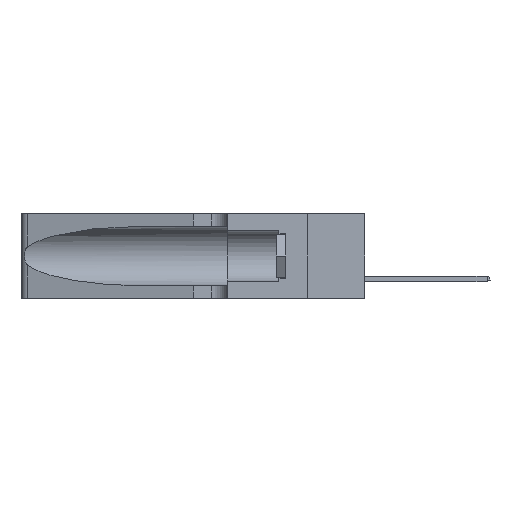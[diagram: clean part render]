
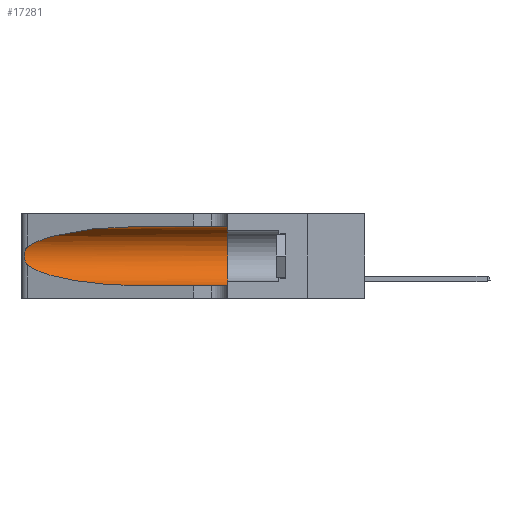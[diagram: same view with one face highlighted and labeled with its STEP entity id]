
A CAD part, left-side view. The second image highlights one B-rep face of the part: STEP entity #17281.
In plain terms, the highlighted cylindrical face has radius 3.308 mm (diameter 6.617 mm), a partial arc.
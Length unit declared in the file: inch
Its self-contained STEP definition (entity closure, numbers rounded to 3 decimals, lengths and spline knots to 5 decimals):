
#176 = CARTESIAN_POINT ( 'NONE',  ( 0.1305, 0.35, 0.31525 ) ) ;
#486 = CARTESIAN_POINT ( 'NONE',  ( 0.26075, 1.23896, 0.178 ) ) ;
#702 = DIRECTION ( 'NONE',  ( 0., -1., 0. ) ) ;
#1172 = VERTEX_POINT ( 'NONE', #8161 ) ;
#1395 = DIRECTION ( 'NONE',  ( 0., -1., 0. ) ) ;
#2424 = VERTEX_POINT ( 'NONE', #16003 ) ;
#2912 = CARTESIAN_POINT ( 'NONE',  ( 0.1305, 0.35, 0.185 ) ) ;
#2987 = DIRECTION ( 'NONE',  ( 0., 1., 0. ) ) ;
#3021 = EDGE_LOOP ( 'NONE', ( #21100, #21108, #21686, #7872, #3442, #13311 ) ) ;
#3167 = B_SPLINE_CURVE_WITH_KNOTS ( 'NONE', 3,
 ( #6841, #21973, #16844, #6610, #8393, #9002, #6990, #486, #12153, #18927, #12298, #3888, #5388, #3669 ),
 .UNSPECIFIED., .F., .F.,
 ( 4, 2, 2, 2, 2, 2, 4 ),
 ( 0., 0.00027, 0.00053, 0.00107, 0.0016, 0.00187, 0.00214 ),
 .UNSPECIFIED. ) ;
#3442 = ORIENTED_EDGE ( 'NONE', *, *, #21819, .F. ) ;
#3669 = CARTESIAN_POINT ( 'NONE',  ( 0.25487, 1.22718, 0.14631 ) ) ;
#3676 = LINE ( 'NONE', #10855, #13487 ) ;
#3888 = CARTESIAN_POINT ( 'NONE',  ( 0.25639, 1.23186, 0.15144 ) ) ;
#3994 = CARTESIAN_POINT ( 'NONE',  ( 0.1305, 0.35, 0.05475 ) ) ;
#4437 = CARTESIAN_POINT ( 'NONE',  ( 0.1305, 0.72297, 0.05475 ) ) ;
#5388 = CARTESIAN_POINT ( 'NONE',  ( 0.25555, 1.22993, 0.14849 ) ) ;
#6610 = CARTESIAN_POINT ( 'NONE',  ( 0.25787, 1.23484, 0.2124 ) ) ;
#6841 = CARTESIAN_POINT ( 'NONE',  ( 0.25487, 1.22718, 0.22369 ) ) ;
#6990 = CARTESIAN_POINT ( 'NONE',  ( 0.26075, 1.23896, 0.19203 ) ) ;
#7119 =( BOUNDED_CURVE ( )  B_SPLINE_CURVE ( 3, ( #11892, #20530, #12055, #13369 ),
 .UNSPECIFIED., .F., .F. ) 
 B_SPLINE_CURVE_WITH_KNOTS ( ( 4, 4 ),
 ( 1.5708, 2.84003 ),
 .UNSPECIFIED. ) 
 CURVE ( )  GEOMETRIC_REPRESENTATION_ITEM ( )  RATIONAL_B_SPLINE_CURVE ( ( 1., 0.87, 0.87, 1. ) ) 
 REPRESENTATION_ITEM ( '' )  );
#7872 = ORIENTED_EDGE ( 'NONE', *, *, #10670, .T. ) ;
#8161 = CARTESIAN_POINT ( 'NONE',  ( 0.25487, 1.22718, 0.14631 ) ) ;
#8183 = CARTESIAN_POINT ( 'NONE',  ( 0.1305, 0.72297, 0.05475 ) ) ;
#8306 = CYLINDRICAL_SURFACE ( 'NONE', #20213, 0.13025 ) ;
#8339 = CARTESIAN_POINT ( 'NONE',  ( 0.1305, 1.61858, 0.185 ) ) ;
#8393 = CARTESIAN_POINT ( 'NONE',  ( 0.25854, 1.2359, 0.20912 ) ) ;
#8400 = CARTESIAN_POINT ( 'NONE',  ( 0.1305, 1.61858, 0.31525 ) ) ;
#8554 = AXIS2_PLACEMENT_3D ( 'NONE', #2912, #2987, #9671 ) ;
#8662 = LINE ( 'NONE', #8400, #20664 ) ;
#8857 = FACE_OUTER_BOUND ( 'NONE', #3021, .T. ) ;
#9002 = CARTESIAN_POINT ( 'NONE',  ( 0.26018, 1.23835, 0.19895 ) ) ;
#9671 = DIRECTION ( 'NONE',  ( 0., 0., 1. ) ) ;
#10670 = EDGE_CURVE ( 'NONE', #20775, #20023, #3676, .T. ) ;
#10855 = CARTESIAN_POINT ( 'NONE',  ( 0.1305, 1.61858, 0.05475 ) ) ;
#11100 =( BOUNDED_CURVE ( )  B_SPLINE_CURVE ( 3, ( #18640, #20344, #15214, #8183 ),
 .UNSPECIFIED., .F., .F. ) 
 B_SPLINE_CURVE_WITH_KNOTS ( ( 4, 4 ),
 ( 3.44316, 4.71239 ),
 .UNSPECIFIED. ) 
 CURVE ( )  GEOMETRIC_REPRESENTATION_ITEM ( )  RATIONAL_B_SPLINE_CURVE ( ( 1., 0.87, 0.87, 1. ) ) 
 REPRESENTATION_ITEM ( '' )  );
#11892 = CARTESIAN_POINT ( 'NONE',  ( 0.1305, 0.72297, 0.31525 ) ) ;
#12055 = CARTESIAN_POINT ( 'NONE',  ( 0.2373, 1.15595, 0.28018 ) ) ;
#12153 = CARTESIAN_POINT ( 'NONE',  ( 0.26017, 1.23833, 0.17102 ) ) ;
#12212 = VERTEX_POINT ( 'NONE', #176 ) ;
#12298 = CARTESIAN_POINT ( 'NONE',  ( 0.25789, 1.23486, 0.15765 ) ) ;
#12636 = CIRCLE ( 'NONE', #8554, 0.13025 ) ;
#13311 = ORIENTED_EDGE ( 'NONE', *, *, #19849, .F. ) ;
#13369 = CARTESIAN_POINT ( 'NONE',  ( 0.25487, 1.22718, 0.22369 ) ) ;
#13487 = VECTOR ( 'NONE', #702, 39.37008 ) ;
#14912 = VERTEX_POINT ( 'NONE', #18455 ) ;
#15214 = CARTESIAN_POINT ( 'NONE',  ( 0.18966, 0.96281, 0.05475 ) ) ;
#16003 = CARTESIAN_POINT ( 'NONE',  ( 0.25487, 1.22718, 0.22369 ) ) ;
#16183 = EDGE_CURVE ( 'NONE', #14912, #2424, #7119, .T. ) ;
#16844 = CARTESIAN_POINT ( 'NONE',  ( 0.25639, 1.23184, 0.21858 ) ) ;
#17281 = ADVANCED_FACE ( 'NONE', ( #8857 ), #8306, .F. ) ;
#17778 = EDGE_CURVE ( 'NONE', #2424, #1172, #3167, .T. ) ;
#18272 = EDGE_CURVE ( 'NONE', #1172, #20775, #11100, .T. ) ;
#18455 = CARTESIAN_POINT ( 'NONE',  ( 0.1305, 0.72297, 0.31525 ) ) ;
#18640 = CARTESIAN_POINT ( 'NONE',  ( 0.25487, 1.22718, 0.14631 ) ) ;
#18927 = CARTESIAN_POINT ( 'NONE',  ( 0.25856, 1.23593, 0.16098 ) ) ;
#19849 = EDGE_CURVE ( 'NONE', #14912, #12212, #8662, .T. ) ;
#20023 = VERTEX_POINT ( 'NONE', #3994 ) ;
#20213 = AXIS2_PLACEMENT_3D ( 'NONE', #8339, #1395, #22064 ) ;
#20344 = CARTESIAN_POINT ( 'NONE',  ( 0.2373, 1.15595, 0.08982 ) ) ;
#20530 = CARTESIAN_POINT ( 'NONE',  ( 0.18966, 0.96281, 0.31525 ) ) ;
#20664 = VECTOR ( 'NONE', #21839, 39.37008 ) ;
#20775 = VERTEX_POINT ( 'NONE', #4437 ) ;
#21100 = ORIENTED_EDGE ( 'NONE', *, *, #16183, .T. ) ;
#21108 = ORIENTED_EDGE ( 'NONE', *, *, #17778, .T. ) ;
#21686 = ORIENTED_EDGE ( 'NONE', *, *, #18272, .T. ) ;
#21819 = EDGE_CURVE ( 'NONE', #12212, #20023, #12636, .T. ) ;
#21839 = DIRECTION ( 'NONE',  ( 0., -1., 0. ) ) ;
#21973 = CARTESIAN_POINT ( 'NONE',  ( 0.25555, 1.22994, 0.2215 ) ) ;
#22064 = DIRECTION ( 'NONE',  ( 0., 0., -1. ) ) ;
